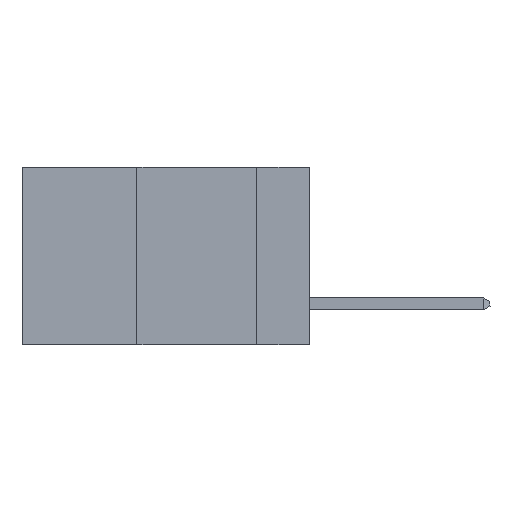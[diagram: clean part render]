
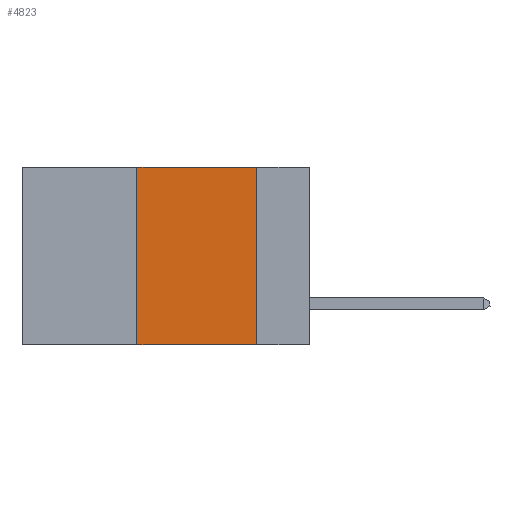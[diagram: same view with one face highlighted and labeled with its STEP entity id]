
A CAD part, left-side view. The second image highlights one B-rep face of the part: STEP entity #4823.
In plain terms, the highlighted planar face has unit normal (-1, 0, 0).
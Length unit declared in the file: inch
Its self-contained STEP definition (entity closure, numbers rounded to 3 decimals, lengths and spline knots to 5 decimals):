
#2568 = CARTESIAN_POINT ( 'NONE',  ( 0., 0.6, 0. ) ) ;
#4634 = DIRECTION ( 'NONE',  ( 1., 0., 0. ) ) ;
#4823 = ADVANCED_FACE ( 'NONE', ( #17519 ), #35342, .F. ) ;
#5058 = LINE ( 'NONE', #27114, #21418 ) ;
#5158 = LINE ( 'NONE', #34343, #12459 ) ;
#6429 = CARTESIAN_POINT ( 'NONE',  ( 0., 0.11, 0. ) ) ;
#7517 = LINE ( 'NONE', #2568, #39035 ) ;
#10042 = EDGE_CURVE ( 'NONE', #30349, #34531, #7517, .T. ) ;
#10680 = EDGE_CURVE ( 'NONE', #18179, #23398, #5058, .T. ) ;
#10936 = CARTESIAN_POINT ( 'NONE',  ( 0., 0.6, 0. ) ) ;
#11708 = ORIENTED_EDGE ( 'NONE', *, *, #27072, .F. ) ;
#12459 = VECTOR ( 'NONE', #37407, 39.37008 ) ;
#16250 = ORIENTED_EDGE ( 'NONE', *, *, #18086, .F. ) ;
#17519 = FACE_OUTER_BOUND ( 'NONE', #33879, .T. ) ;
#18086 = EDGE_CURVE ( 'NONE', #18179, #30349, #5158, .T. ) ;
#18179 = VERTEX_POINT ( 'NONE', #37936 ) ;
#18335 = VECTOR ( 'NONE', #37455, 39.37008 ) ;
#21128 = CARTESIAN_POINT ( 'NONE',  ( 0., 0.36, 0. ) ) ;
#21418 = VECTOR ( 'NONE', #30149, 39.37008 ) ;
#23398 = VERTEX_POINT ( 'NONE', #34835 ) ;
#27072 = EDGE_CURVE ( 'NONE', #34531, #23398, #33626, .T. ) ;
#27114 = CARTESIAN_POINT ( 'NONE',  ( 0., 0.6, -0.37 ) ) ;
#27291 = DIRECTION ( 'NONE',  ( 0., -1., 0. ) ) ;
#28188 = ORIENTED_EDGE ( 'NONE', *, *, #10042, .F. ) ;
#30149 = DIRECTION ( 'NONE',  ( 0., -1., 0. ) ) ;
#30349 = VERTEX_POINT ( 'NONE', #21128 ) ;
#33388 = AXIS2_PLACEMENT_3D ( 'NONE', #10936, #4634, #38383 ) ;
#33626 = LINE ( 'NONE', #34395, #18335 ) ;
#33879 = EDGE_LOOP ( 'NONE', ( #11708, #28188, #16250, #36390 ) ) ;
#34343 = CARTESIAN_POINT ( 'NONE',  ( 0., 0.36, 0. ) ) ;
#34395 = CARTESIAN_POINT ( 'NONE',  ( 0., 0.11, 0. ) ) ;
#34531 = VERTEX_POINT ( 'NONE', #6429 ) ;
#34835 = CARTESIAN_POINT ( 'NONE',  ( 0., 0.11, -0.37 ) ) ;
#35342 = PLANE ( 'NONE',  #33388 ) ;
#36390 = ORIENTED_EDGE ( 'NONE', *, *, #10680, .T. ) ;
#37407 = DIRECTION ( 'NONE',  ( 0., 0., 1. ) ) ;
#37455 = DIRECTION ( 'NONE',  ( 0., 0., -1. ) ) ;
#37936 = CARTESIAN_POINT ( 'NONE',  ( 0., 0.36, -0.37 ) ) ;
#38383 = DIRECTION ( 'NONE',  ( 0., 0., -1. ) ) ;
#39035 = VECTOR ( 'NONE', #27291, 39.37008 ) ;
